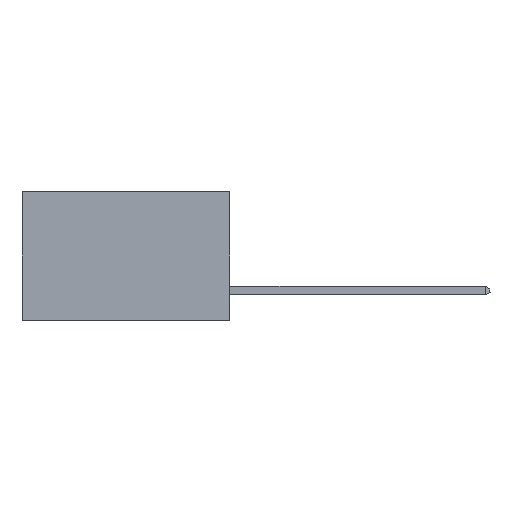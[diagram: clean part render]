
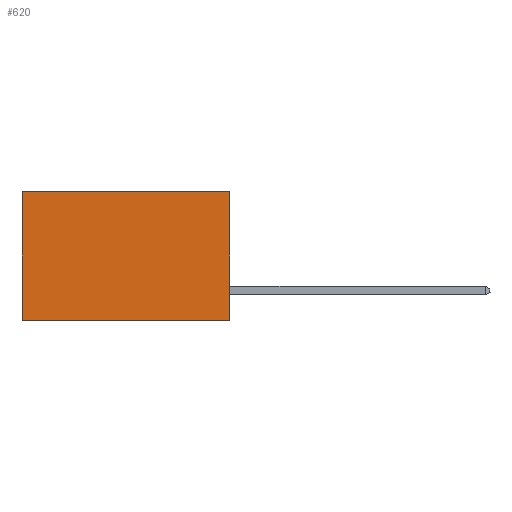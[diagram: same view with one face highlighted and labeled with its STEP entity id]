
A CAD part, left-side view. The second image highlights one B-rep face of the part: STEP entity #620.
In plain terms, the highlighted planar face has unit normal (-1, 0, 0).
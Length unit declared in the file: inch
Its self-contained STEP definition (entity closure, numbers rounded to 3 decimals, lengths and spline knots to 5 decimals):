
#91 = CARTESIAN_POINT ( 'NONE',  ( 0.298, 0., 0. ) ) ;
#518 = EDGE_CURVE ( 'NONE', #1721, #5825, #9568, .T. ) ;
#620 = ADVANCED_FACE ( 'NONE', ( #1190 ), #7746, .F. ) ;
#646 = VECTOR ( 'NONE', #13031, 39.37008 ) ;
#828 = CARTESIAN_POINT ( 'NONE',  ( 0.298, 0.6, -0.37 ) ) ;
#1190 = FACE_OUTER_BOUND ( 'NONE', #4109, .T. ) ;
#1721 = VERTEX_POINT ( 'NONE', #11154 ) ;
#2351 = CARTESIAN_POINT ( 'NONE',  ( 0.298, 0., -0.37 ) ) ;
#3582 = ORIENTED_EDGE ( 'NONE', *, *, #518, .T. ) ;
#3771 = ORIENTED_EDGE ( 'NONE', *, *, #9072, .F. ) ;
#4109 = EDGE_LOOP ( 'NONE', ( #6332, #4667, #3771, #3582 ) ) ;
#4667 = ORIENTED_EDGE ( 'NONE', *, *, #10680, .F. ) ;
#4801 = DIRECTION ( 'NONE',  ( 1., 0., 0. ) ) ;
#5560 = CARTESIAN_POINT ( 'NONE',  ( 0.298, 0.6, 0. ) ) ;
#5825 = VERTEX_POINT ( 'NONE', #5560 ) ;
#6124 = CARTESIAN_POINT ( 'NONE',  ( 0.298, 0., -0.37 ) ) ;
#6332 = ORIENTED_EDGE ( 'NONE', *, *, #11332, .T. ) ;
#7682 = VECTOR ( 'NONE', #12515, 39.37008 ) ;
#7746 = PLANE ( 'NONE',  #9961 ) ;
#9062 = DIRECTION ( 'NONE',  ( 0., 0., -1. ) ) ;
#9072 = EDGE_CURVE ( 'NONE', #1721, #9749, #9907, .T. ) ;
#9183 = CARTESIAN_POINT ( 'NONE',  ( 0.298, 0.6, 0. ) ) ;
#9428 = DIRECTION ( 'NONE',  ( 0., 0., -1. ) ) ;
#9568 = LINE ( 'NONE', #10860, #9880 ) ;
#9749 = VERTEX_POINT ( 'NONE', #2351 ) ;
#9880 = VECTOR ( 'NONE', #11904, 39.37008 ) ;
#9907 = LINE ( 'NONE', #91, #12015 ) ;
#9961 = AXIS2_PLACEMENT_3D ( 'NONE', #11755, #4801, #9062 ) ;
#10484 = LINE ( 'NONE', #6124, #7682 ) ;
#10680 = EDGE_CURVE ( 'NONE', #9749, #13151, #10484, .T. ) ;
#10860 = CARTESIAN_POINT ( 'NONE',  ( 0.298, 0., 0. ) ) ;
#11154 = CARTESIAN_POINT ( 'NONE',  ( 0.298, 0., 0. ) ) ;
#11332 = EDGE_CURVE ( 'NONE', #5825, #13151, #13424, .T. ) ;
#11755 = CARTESIAN_POINT ( 'NONE',  ( 0.298, 0., 0. ) ) ;
#11904 = DIRECTION ( 'NONE',  ( 0., 1., 0. ) ) ;
#12015 = VECTOR ( 'NONE', #9428, 39.37008 ) ;
#12515 = DIRECTION ( 'NONE',  ( 0., 1., 0. ) ) ;
#13031 = DIRECTION ( 'NONE',  ( 0., 0., -1. ) ) ;
#13151 = VERTEX_POINT ( 'NONE', #828 ) ;
#13424 = LINE ( 'NONE', #9183, #646 ) ;
